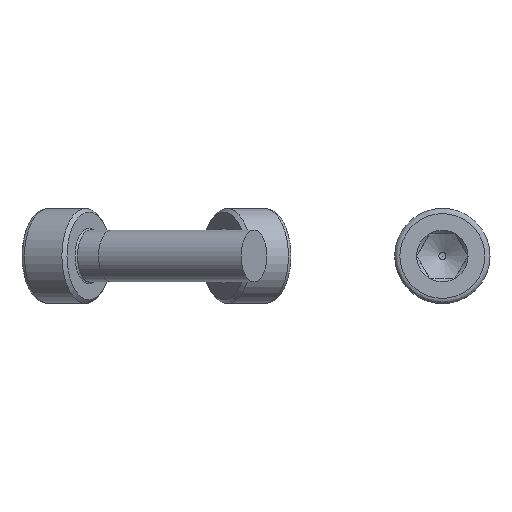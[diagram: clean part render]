
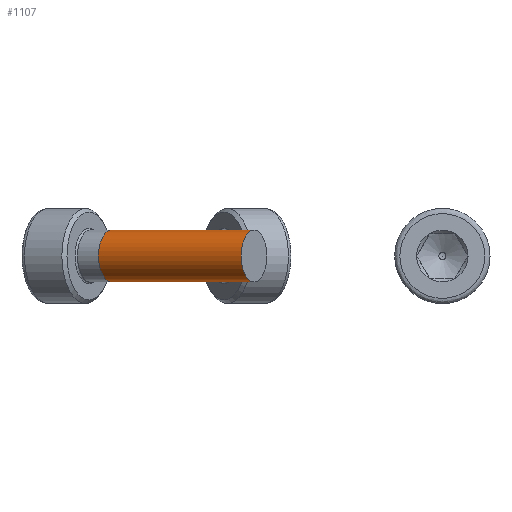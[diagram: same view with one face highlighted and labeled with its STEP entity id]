
A CAD part, front view. The second image highlights one B-rep face of the part: STEP entity #1107.
In plain terms, the highlighted cylindrical face has radius 1.5 mm (diameter 3 mm), a full revolution.
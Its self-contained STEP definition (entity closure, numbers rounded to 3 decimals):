
#1040 = CYLINDRICAL_SURFACE('',#1041,1.5);
#1041 = AXIS2_PLACEMENT_3D('',#1042,#1043,#1044);
#1042 = CARTESIAN_POINT('',(-9.311,-7.326,23.));
#1043 = DIRECTION('',(0.866,-0.5,-0.));
#1044 = DIRECTION('',(-0.5,-0.866,0.));
#1058 = VERTEX_POINT('',#1059);
#1059 = CARTESIAN_POINT('',(-8.848,-9.325,23.));
#1080 = EDGE_CURVE('',#1058,#1058,#1081,.T.);
#1081 = SURFACE_CURVE('',#1082,(#1087,#1094),.PCURVE_S1.);
#1082 = CIRCLE('',#1083,1.5);
#1083 = AXIS2_PLACEMENT_3D('',#1084,#1085,#1086);
#1084 = CARTESIAN_POINT('',(-8.098,-8.026,23.));
#1085 = DIRECTION('',(-0.866,0.5,0.));
#1086 = DIRECTION('',(-0.5,-0.866,0.));
#1087 = PCURVE('',#1040,#1088);
#1088 = DEFINITIONAL_REPRESENTATION('',(#1089),#1093);
#1089 = LINE('',#1090,#1091);
#1090 = CARTESIAN_POINT('',(-0.,1.4));
#1091 = VECTOR('',#1092,1.);
#1092 = DIRECTION('',(-1.,0.));
#1093 = ( GEOMETRIC_REPRESENTATION_CONTEXT(2) 
PARAMETRIC_REPRESENTATION_CONTEXT() REPRESENTATION_CONTEXT('2D SPACE',''
  ) );
#1094 = PCURVE('',#1095,#1100);
#1095 = CYLINDRICAL_SURFACE('',#1096,1.5);
#1096 = AXIS2_PLACEMENT_3D('',#1097,#1098,#1099);
#1097 = CARTESIAN_POINT('',(-8.098,-8.026,23.));
#1098 = DIRECTION('',(0.866,-0.5,-0.));
#1099 = DIRECTION('',(-0.5,-0.866,0.));
#1100 = DEFINITIONAL_REPRESENTATION('',(#1101),#1105);
#1101 = LINE('',#1102,#1103);
#1102 = CARTESIAN_POINT('',(-0.,0.));
#1103 = VECTOR('',#1104,1.);
#1104 = DIRECTION('',(-1.,0.));
#1105 = ( GEOMETRIC_REPRESENTATION_CONTEXT(2) 
PARAMETRIC_REPRESENTATION_CONTEXT() REPRESENTATION_CONTEXT('2D SPACE',''
  ) );
#1107 = ADVANCED_FACE('',(#1108),#1095,.T.);
#1108 = FACE_BOUND('',#1109,.F.);
#1109 = EDGE_LOOP('',(#1110,#1133,#1134,#1135));
#1110 = ORIENTED_EDGE('',*,*,#1111,.F.);
#1111 = EDGE_CURVE('',#1058,#1112,#1114,.T.);
#1112 = VERTEX_POINT('',#1113);
#1113 = CARTESIAN_POINT('',(-0.621,-14.075,23.));
#1114 = SEAM_CURVE('',#1115,(#1119,#1126),.PCURVE_S1.);
#1115 = LINE('',#1116,#1117);
#1116 = CARTESIAN_POINT('',(-8.848,-9.325,23.));
#1117 = VECTOR('',#1118,1.);
#1118 = DIRECTION('',(0.866,-0.5,0.));
#1119 = PCURVE('',#1095,#1120);
#1120 = DEFINITIONAL_REPRESENTATION('',(#1121),#1125);
#1121 = LINE('',#1122,#1123);
#1122 = CARTESIAN_POINT('',(-0.,0.));
#1123 = VECTOR('',#1124,1.);
#1124 = DIRECTION('',(-0.,1.));
#1125 = ( GEOMETRIC_REPRESENTATION_CONTEXT(2) 
PARAMETRIC_REPRESENTATION_CONTEXT() REPRESENTATION_CONTEXT('2D SPACE',''
  ) );
#1126 = PCURVE('',#1095,#1127);
#1127 = DEFINITIONAL_REPRESENTATION('',(#1128),#1132);
#1128 = LINE('',#1129,#1130);
#1129 = CARTESIAN_POINT('',(-6.283,0.));
#1130 = VECTOR('',#1131,1.);
#1131 = DIRECTION('',(-0.,1.));
#1132 = ( GEOMETRIC_REPRESENTATION_CONTEXT(2) 
PARAMETRIC_REPRESENTATION_CONTEXT() REPRESENTATION_CONTEXT('2D SPACE',''
  ) );
#1133 = ORIENTED_EDGE('',*,*,#1080,.T.);
#1134 = ORIENTED_EDGE('',*,*,#1111,.T.);
#1135 = ORIENTED_EDGE('',*,*,#1136,.T.);
#1136 = EDGE_CURVE('',#1112,#1112,#1137,.T.);
#1137 = SURFACE_CURVE('',#1138,(#1143,#1150),.PCURVE_S1.);
#1138 = CIRCLE('',#1139,1.5);
#1139 = AXIS2_PLACEMENT_3D('',#1140,#1141,#1142);
#1140 = CARTESIAN_POINT('',(0.129,-12.776,23.));
#1141 = DIRECTION('',(0.866,-0.5,0.));
#1142 = DIRECTION('',(-0.5,-0.866,0.));
#1143 = PCURVE('',#1095,#1144);
#1144 = DEFINITIONAL_REPRESENTATION('',(#1145),#1149);
#1145 = LINE('',#1146,#1147);
#1146 = CARTESIAN_POINT('',(-6.283,9.5));
#1147 = VECTOR('',#1148,1.);
#1148 = DIRECTION('',(1.,-0.));
#1149 = ( GEOMETRIC_REPRESENTATION_CONTEXT(2) 
PARAMETRIC_REPRESENTATION_CONTEXT() REPRESENTATION_CONTEXT('2D SPACE',''
  ) );
#1150 = PCURVE('',#1151,#1156);
#1151 = PLANE('',#1152);
#1152 = AXIS2_PLACEMENT_3D('',#1153,#1154,#1155);
#1153 = CARTESIAN_POINT('',(3.129,-7.58,17.));
#1154 = DIRECTION('',(0.866,-0.5,0.));
#1155 = DIRECTION('',(0.,0.,1.));
#1156 = DEFINITIONAL_REPRESENTATION('',(#1157),#1161);
#1157 = CIRCLE('',#1158,1.5);
#1158 = AXIS2_PLACEMENT_2D('',#1159,#1160);
#1159 = CARTESIAN_POINT('',(6.,6.));
#1160 = DIRECTION('',(0.,1.));
#1161 = ( GEOMETRIC_REPRESENTATION_CONTEXT(2) 
PARAMETRIC_REPRESENTATION_CONTEXT() REPRESENTATION_CONTEXT('2D SPACE',''
  ) );
